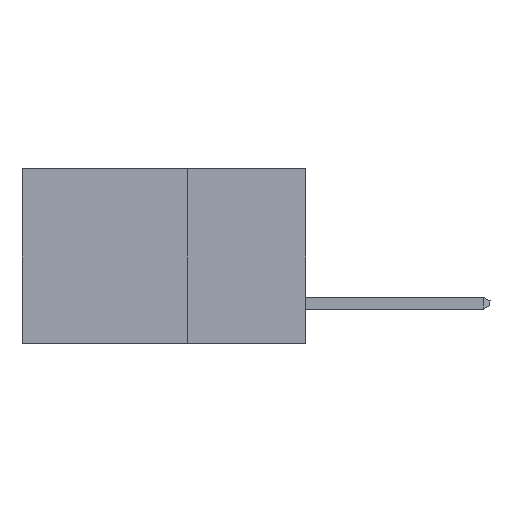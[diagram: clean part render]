
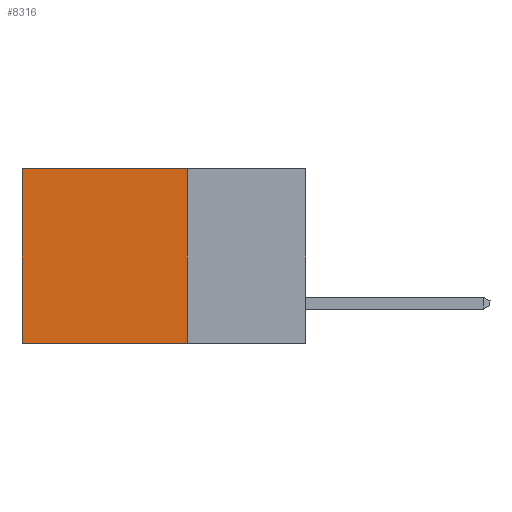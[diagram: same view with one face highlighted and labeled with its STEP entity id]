
A CAD part, left-side view. The second image highlights one B-rep face of the part: STEP entity #8316.
In plain terms, the highlighted planar face has unit normal (-1, 0, 0).
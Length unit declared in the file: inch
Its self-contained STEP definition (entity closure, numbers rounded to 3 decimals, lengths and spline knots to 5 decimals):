
#179 = FACE_OUTER_BOUND ( 'NONE', #2817, .T. ) ;
#195 = VERTEX_POINT ( 'NONE', #6909 ) ;
#711 = EDGE_CURVE ( 'NONE', #4039, #8512, #11450, .T. ) ;
#1161 = VECTOR ( 'NONE', #7097, 39.37008 ) ;
#1947 = CARTESIAN_POINT ( 'NONE',  ( 0.2615, 0.25, 0. ) ) ;
#2653 = VECTOR ( 'NONE', #4171, 39.37008 ) ;
#2817 = EDGE_LOOP ( 'NONE', ( #11782, #7122, #8777, #6166 ) ) ;
#3416 = CARTESIAN_POINT ( 'NONE',  ( 0.2615, 0.25, -0.37 ) ) ;
#3816 = CARTESIAN_POINT ( 'NONE',  ( 0.2615, 0.6, 0. ) ) ;
#4025 = EDGE_CURVE ( 'NONE', #195, #7178, #11240, .T. ) ;
#4039 = VERTEX_POINT ( 'NONE', #1947 ) ;
#4167 = CARTESIAN_POINT ( 'NONE',  ( 0.2615, 0.25, -0.37 ) ) ;
#4171 = DIRECTION ( 'NONE',  ( 0., 1., 0. ) ) ;
#4429 = CARTESIAN_POINT ( 'NONE',  ( 0.2615, 0.6, -0.37 ) ) ;
#4729 = EDGE_CURVE ( 'NONE', #4039, #195, #5718, .T. ) ;
#5094 = EDGE_CURVE ( 'NONE', #8512, #7178, #7278, .T. ) ;
#5535 = AXIS2_PLACEMENT_3D ( 'NONE', #4167, #7228, #7302 ) ;
#5641 = DIRECTION ( 'NONE',  ( 0., 0., -1. ) ) ;
#5718 = LINE ( 'NONE', #3416, #6350 ) ;
#6166 = ORIENTED_EDGE ( 'NONE', *, *, #711, .T. ) ;
#6317 = CARTESIAN_POINT ( 'NONE',  ( 0.2615, 0.6, -0.37 ) ) ;
#6350 = VECTOR ( 'NONE', #5641, 39.37008 ) ;
#6909 = CARTESIAN_POINT ( 'NONE',  ( 0.2615, 0.25, -0.37 ) ) ;
#7097 = DIRECTION ( 'NONE',  ( 0., 1., 0. ) ) ;
#7122 = ORIENTED_EDGE ( 'NONE', *, *, #4025, .F. ) ;
#7178 = VERTEX_POINT ( 'NONE', #4429 ) ;
#7228 = DIRECTION ( 'NONE',  ( 1., 0., 0. ) ) ;
#7278 = LINE ( 'NONE', #6317, #8535 ) ;
#7302 = DIRECTION ( 'NONE',  ( 0., 0., -1. ) ) ;
#7308 = CARTESIAN_POINT ( 'NONE',  ( 0.2615, 0.25, 0. ) ) ;
#8316 = ADVANCED_FACE ( 'NONE', ( #179 ), #12527, .F. ) ;
#8512 = VERTEX_POINT ( 'NONE', #3816 ) ;
#8535 = VECTOR ( 'NONE', #11422, 39.37008 ) ;
#8777 = ORIENTED_EDGE ( 'NONE', *, *, #4729, .F. ) ;
#11240 = LINE ( 'NONE', #13273, #1161 ) ;
#11422 = DIRECTION ( 'NONE',  ( 0., 0., -1. ) ) ;
#11450 = LINE ( 'NONE', #7308, #2653 ) ;
#11782 = ORIENTED_EDGE ( 'NONE', *, *, #5094, .T. ) ;
#12527 = PLANE ( 'NONE',  #5535 ) ;
#13273 = CARTESIAN_POINT ( 'NONE',  ( 0.2615, 0.25, -0.37 ) ) ;
